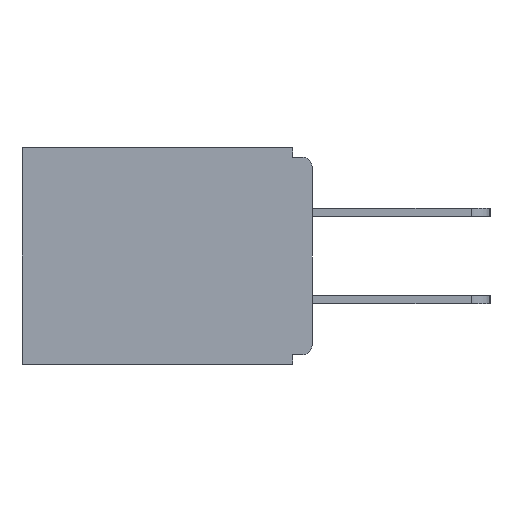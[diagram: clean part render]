
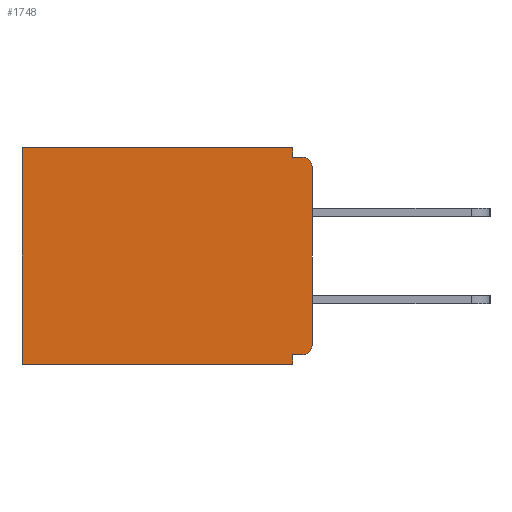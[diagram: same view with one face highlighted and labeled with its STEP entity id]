
A CAD part, left-side view. The second image highlights one B-rep face of the part: STEP entity #1748.
In plain terms, the highlighted planar face has unit normal (-1, 0, 0).
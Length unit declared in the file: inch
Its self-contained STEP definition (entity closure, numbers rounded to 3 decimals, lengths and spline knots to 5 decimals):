
#204 = CARTESIAN_POINT ( 'NONE',  ( 0.298, 0., -0.313 ) ) ;
#570 = ORIENTED_EDGE ( 'NONE', *, *, #964, .F. ) ;
#923 = LINE ( 'NONE', #3118, #18841 ) ;
#964 = EDGE_CURVE ( 'NONE', #8551, #5997, #13267, .T. ) ;
#1408 = CARTESIAN_POINT ( 'NONE',  ( 0.298, 0., -0.343 ) ) ;
#1601 = EDGE_CURVE ( 'NONE', #8551, #6960, #2030, .T. ) ;
#1748 = ADVANCED_FACE ( 'NONE', ( #10958 ), #11265, .F. ) ;
#1964 = DIRECTION ( 'NONE',  ( 0., 0., -1. ) ) ;
#2030 = CIRCLE ( 'NONE', #11572, 0.015 ) ;
#2457 = CARTESIAN_POINT ( 'NONE',  ( 0.298, 0.46, -0.343 ) ) ;
#2459 = ORIENTED_EDGE ( 'NONE', *, *, #12485, .F. ) ;
#2848 = CARTESIAN_POINT ( 'NONE',  ( 0.298, 0.031, -0.015 ) ) ;
#3118 = CARTESIAN_POINT ( 'NONE',  ( 0.298, 0.031, -0.343 ) ) ;
#3759 = EDGE_CURVE ( 'NONE', #15029, #4300, #4332, .T. ) ;
#4273 = EDGE_CURVE ( 'NONE', #5353, #9922, #18996, .T. ) ;
#4300 = VERTEX_POINT ( 'NONE', #2457 ) ;
#4332 = LINE ( 'NONE', #1408, #17177 ) ;
#4568 = ORIENTED_EDGE ( 'NONE', *, *, #4273, .T. ) ;
#5034 = CARTESIAN_POINT ( 'NONE',  ( 0.298, 0.46, 0. ) ) ;
#5094 = VECTOR ( 'NONE', #10406, 39.37008 ) ;
#5353 = VERTEX_POINT ( 'NONE', #6410 ) ;
#5398 = ORIENTED_EDGE ( 'NONE', *, *, #8446, .F. ) ;
#5433 = CARTESIAN_POINT ( 'NONE',  ( 0.298, 0., -0.328 ) ) ;
#5997 = VERTEX_POINT ( 'NONE', #204 ) ;
#6054 = AXIS2_PLACEMENT_3D ( 'NONE', #17703, #8905, #11837 ) ;
#6375 = ORIENTED_EDGE ( 'NONE', *, *, #13598, .F. ) ;
#6400 = EDGE_LOOP ( 'NONE', ( #10166, #5398, #2459, #4568, #9497, #13719, #6375, #7960, #7886, #570 ) ) ;
#6410 = CARTESIAN_POINT ( 'NONE',  ( 0.298, 0.031, 0. ) ) ;
#6424 = VERTEX_POINT ( 'NONE', #15786 ) ;
#6631 = DIRECTION ( 'NONE',  ( 0., 0., -1. ) ) ;
#6827 = DIRECTION ( 'NONE',  ( 1., 0., 0. ) ) ;
#6912 = DIRECTION ( 'NONE',  ( 0., 1., 0. ) ) ;
#6960 = VERTEX_POINT ( 'NONE', #8100 ) ;
#7005 = CARTESIAN_POINT ( 'NONE',  ( 0.298, 0., 0. ) ) ;
#7113 = DIRECTION ( 'NONE',  ( 0., -1., 0. ) ) ;
#7331 = LINE ( 'NONE', #5433, #15933 ) ;
#7555 = EDGE_CURVE ( 'NONE', #9922, #4300, #9358, .T. ) ;
#7886 = ORIENTED_EDGE ( 'NONE', *, *, #12098, .T. ) ;
#7960 = ORIENTED_EDGE ( 'NONE', *, *, #10507, .F. ) ;
#8100 = CARTESIAN_POINT ( 'NONE',  ( 0.298, 0.015, -0.015 ) ) ;
#8407 = VECTOR ( 'NONE', #6631, 39.37008 ) ;
#8446 = EDGE_CURVE ( 'NONE', #16374, #6960, #11845, .T. ) ;
#8551 = VERTEX_POINT ( 'NONE', #14572 ) ;
#8905 = DIRECTION ( 'NONE',  ( -1., 0., 0. ) ) ;
#9358 = LINE ( 'NONE', #5034, #8407 ) ;
#9497 = ORIENTED_EDGE ( 'NONE', *, *, #7555, .T. ) ;
#9865 = CIRCLE ( 'NONE', #6054, 0.015 ) ;
#9922 = VERTEX_POINT ( 'NONE', #17821 ) ;
#10166 = ORIENTED_EDGE ( 'NONE', *, *, #1601, .T. ) ;
#10406 = DIRECTION ( 'NONE',  ( 0., 0., -1. ) ) ;
#10507 = EDGE_CURVE ( 'NONE', #6424, #12919, #7331, .T. ) ;
#10958 = FACE_OUTER_BOUND ( 'NONE', #6400, .T. ) ;
#11026 = DIRECTION ( 'NONE',  ( -1., 0., 0. ) ) ;
#11151 = DIRECTION ( 'NONE',  ( 0., 0., -1. ) ) ;
#11251 = CARTESIAN_POINT ( 'NONE',  ( 0.298, 0., 0. ) ) ;
#11265 = PLANE ( 'NONE',  #13547 ) ;
#11391 = CARTESIAN_POINT ( 'NONE',  ( 0.298, 0.031, -0.328 ) ) ;
#11572 = AXIS2_PLACEMENT_3D ( 'NONE', #18094, #11026, #1964 ) ;
#11837 = DIRECTION ( 'NONE',  ( 0., 0., -1. ) ) ;
#11845 = LINE ( 'NONE', #17236, #15563 ) ;
#12098 = EDGE_CURVE ( 'NONE', #6424, #5997, #9865, .T. ) ;
#12122 = VECTOR ( 'NONE', #18855, 39.37008 ) ;
#12485 = EDGE_CURVE ( 'NONE', #5353, #16374, #923, .T. ) ;
#12761 = VECTOR ( 'NONE', #15847, 39.37008 ) ;
#12919 = VERTEX_POINT ( 'NONE', #11391 ) ;
#13267 = LINE ( 'NONE', #11251, #12122 ) ;
#13547 = AXIS2_PLACEMENT_3D ( 'NONE', #14221, #6827, #11151 ) ;
#13598 = EDGE_CURVE ( 'NONE', #12919, #15029, #18586, .T. ) ;
#13719 = ORIENTED_EDGE ( 'NONE', *, *, #3759, .F. ) ;
#14221 = CARTESIAN_POINT ( 'NONE',  ( 0.298, 0., 0. ) ) ;
#14572 = CARTESIAN_POINT ( 'NONE',  ( 0.298, 0., -0.03 ) ) ;
#15029 = VERTEX_POINT ( 'NONE', #16917 ) ;
#15563 = VECTOR ( 'NONE', #7113, 39.37008 ) ;
#15786 = CARTESIAN_POINT ( 'NONE',  ( 0.298, 0.015, -0.328 ) ) ;
#15847 = DIRECTION ( 'NONE',  ( 0., 1., 0. ) ) ;
#15933 = VECTOR ( 'NONE', #6912, 39.37008 ) ;
#16276 = CARTESIAN_POINT ( 'NONE',  ( 0.298, 0.031, -0.343 ) ) ;
#16374 = VERTEX_POINT ( 'NONE', #2848 ) ;
#16917 = CARTESIAN_POINT ( 'NONE',  ( 0.298, 0.031, -0.343 ) ) ;
#17177 = VECTOR ( 'NONE', #17993, 39.37008 ) ;
#17236 = CARTESIAN_POINT ( 'NONE',  ( 0.298, 0., -0.015 ) ) ;
#17703 = CARTESIAN_POINT ( 'NONE',  ( 0.298, 0.015, -0.313 ) ) ;
#17778 = DIRECTION ( 'NONE',  ( 0., 0., -1. ) ) ;
#17821 = CARTESIAN_POINT ( 'NONE',  ( 0.298, 0.46, 0. ) ) ;
#17993 = DIRECTION ( 'NONE',  ( 0., 1., 0. ) ) ;
#18094 = CARTESIAN_POINT ( 'NONE',  ( 0.298, 0.015, -0.03 ) ) ;
#18586 = LINE ( 'NONE', #16276, #5094 ) ;
#18841 = VECTOR ( 'NONE', #17778, 39.37008 ) ;
#18855 = DIRECTION ( 'NONE',  ( 0., 0., -1. ) ) ;
#18996 = LINE ( 'NONE', #7005, #12761 ) ;
